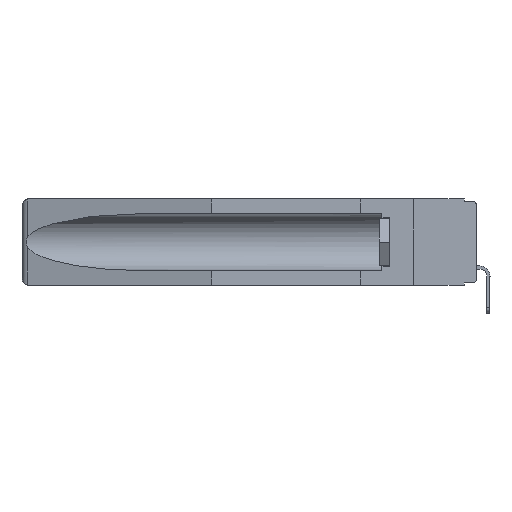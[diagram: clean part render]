
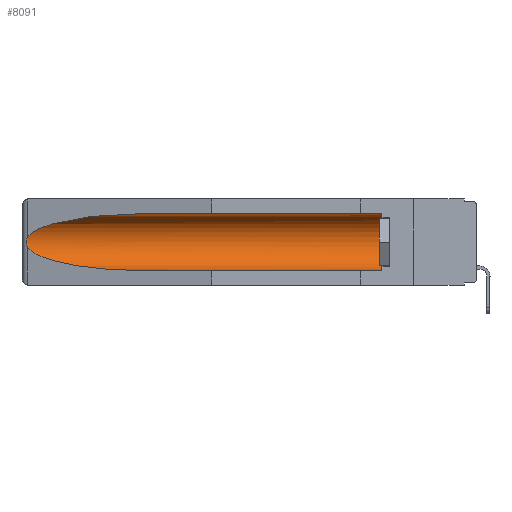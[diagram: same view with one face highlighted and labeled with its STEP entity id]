
A CAD part, left-side view. The second image highlights one B-rep face of the part: STEP entity #8091.
In plain terms, the highlighted cylindrical face has radius 2.857 mm (diameter 5.715 mm), a partial arc.
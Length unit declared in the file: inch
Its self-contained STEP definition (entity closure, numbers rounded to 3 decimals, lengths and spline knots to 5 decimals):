
#86 = CARTESIAN_POINT ( 'NONE',  ( 0.26537, 1.52718, -0.14972 ) ) ;
#136 = CARTESIAN_POINT ( 'NONE',  ( 0.2673, 1.5327, -0.16383 ) ) ;
#172 = EDGE_CURVE ( 'NONE', #9058, #12660, #3271, .T. ) ;
#1187 = DIRECTION ( 'NONE',  ( 0., 1., 0. ) ) ;
#1372 = DIRECTION ( 'NONE',  ( 0., 1., 0. ) ) ;
#1738 = CARTESIAN_POINT ( 'NONE',  ( 0.2673, 1.53269, -0.17917 ) ) ;
#1759 = ORIENTED_EDGE ( 'NONE', *, *, #14701, .T. ) ;
#1830 = CARTESIAN_POINT ( 'NONE',  ( 0.26654, 1.53092, -0.15636 ) ) ;
#1890 = CARTESIAN_POINT ( 'NONE',  ( 0.21114, 1.30732, -0.284 ) ) ;
#2155 = LINE ( 'NONE', #8612, #16605 ) ;
#2253 = EDGE_LOOP ( 'NONE', ( #1759, #11903, #10346, #12034, #5680, #13302 ) ) ;
#2475 = CARTESIAN_POINT ( 'NONE',  ( 0.155, -0.30754, -0.1715 ) ) ;
#3074 = EDGE_CURVE ( 'NONE', #16322, #10199, #15776, .T. ) ;
#3271 = LINE ( 'NONE', #19186, #10555 ) ;
#4268 = CARTESIAN_POINT ( 'NONE',  ( 0.155, 0.126, -0.1715 ) ) ;
#4823 = CARTESIAN_POINT ( 'NONE',  ( 0.26537, 1.52718, -0.19328 ) ) ;
#5309 = CARTESIAN_POINT ( 'NONE',  ( 0.155, 1.07973, -0.059 ) ) ;
#5680 = ORIENTED_EDGE ( 'NONE', *, *, #5923, .T. ) ;
#5923 = EDGE_CURVE ( 'NONE', #13357, #9058, #12169, .T. ) ;
#6426 = CARTESIAN_POINT ( 'NONE',  ( 0.155, 1.07973, -0.284 ) ) ;
#6949 = CARTESIAN_POINT ( 'NONE',  ( 0.155, 0.126, -0.059 ) ) ;
#8091 = ADVANCED_FACE ( 'NONE', ( #18598 ), #10551, .F. ) ;
#8191 = CARTESIAN_POINT ( 'NONE',  ( 0.26655, 1.53094, -0.18657 ) ) ;
#8358 = CARTESIAN_POINT ( 'NONE',  ( 0.155, 1.07973, -0.284 ) ) ;
#8612 = CARTESIAN_POINT ( 'NONE',  ( 0.155, -0.30754, -0.284 ) ) ;
#9058 = VERTEX_POINT ( 'NONE', #6949 ) ;
#9150 = DIRECTION ( 'NONE',  ( 0., 0., 1. ) ) ;
#9908 = CARTESIAN_POINT ( 'NONE',  ( 0.2675, 1.53308, -0.16763 ) ) ;
#10199 = VERTEX_POINT ( 'NONE', #6426 ) ;
#10346 = ORIENTED_EDGE ( 'NONE', *, *, #3074, .T. ) ;
#10551 = CYLINDRICAL_SURFACE ( 'NONE', #20017, 0.1125 ) ;
#10555 = VECTOR ( 'NONE', #1372, 39.37008 ) ;
#11758 = CARTESIAN_POINT ( 'NONE',  ( 0.155, 1.07973, -0.059 ) ) ;
#11903 = ORIENTED_EDGE ( 'NONE', *, *, #19838, .T. ) ;
#12034 = ORIENTED_EDGE ( 'NONE', *, *, #20011, .F. ) ;
#12169 = CIRCLE ( 'NONE', #16913, 0.1125 ) ;
#12452 = DIRECTION ( 'NONE',  ( 0., -1., 0. ) ) ;
#12660 = VERTEX_POINT ( 'NONE', #5309 ) ;
#12694 =( BOUNDED_CURVE ( )  B_SPLINE_CURVE ( 3, ( #11758, #18221, #14652, #86 ),
 .UNSPECIFIED., .F., .F. ) 
 B_SPLINE_CURVE_WITH_KNOTS ( ( 4, 4 ),
 ( 4.71239, 6.08839 ),
 .UNSPECIFIED. ) 
 CURVE ( )  GEOMETRIC_REPRESENTATION_ITEM ( )  RATIONAL_B_SPLINE_CURVE ( ( 1., 0.848, 0.848, 1. ) ) 
 REPRESENTATION_ITEM ( '' )  );
#13019 = CARTESIAN_POINT ( 'NONE',  ( 0.26537, 1.52718, -0.14972 ) ) ;
#13081 = CARTESIAN_POINT ( 'NONE',  ( 0.26537, 1.52718, -0.19328 ) ) ;
#13302 = ORIENTED_EDGE ( 'NONE', *, *, #172, .T. ) ;
#13357 = VERTEX_POINT ( 'NONE', #20550 ) ;
#14055 = DIRECTION ( 'NONE',  ( 0., 0., 1. ) ) ;
#14652 = CARTESIAN_POINT ( 'NONE',  ( 0.25451, 1.48313, -0.09465 ) ) ;
#14701 = EDGE_CURVE ( 'NONE', #12660, #19686, #12694, .T. ) ;
#14705 = CARTESIAN_POINT ( 'NONE',  ( 0.26597, 1.5296, -0.19026 ) ) ;
#14715 = B_SPLINE_CURVE_WITH_KNOTS ( 'NONE', 3,
 ( #13019, #16302, #1830, #136, #9908, #19350, #1738, #8191, #14705, #4823 ),
 .UNSPECIFIED., .F., .F.,
 ( 4, 2, 2, 2, 4 ),
 ( 0., 0.00029, 0.00058, 0.00087, 0.00117 ),
 .UNSPECIFIED. ) ;
#15776 =( BOUNDED_CURVE ( )  B_SPLINE_CURVE ( 3, ( #17558, #16469, #1890, #8358 ),
 .UNSPECIFIED., .F., .F. ) 
 B_SPLINE_CURVE_WITH_KNOTS ( ( 4, 4 ),
 ( 0.1948, 1.5708 ),
 .UNSPECIFIED. ) 
 CURVE ( )  GEOMETRIC_REPRESENTATION_ITEM ( )  RATIONAL_B_SPLINE_CURVE ( ( 1., 0.848, 0.848, 1. ) ) 
 REPRESENTATION_ITEM ( '' )  );
#16302 = CARTESIAN_POINT ( 'NONE',  ( 0.26597, 1.52961, -0.15275 ) ) ;
#16322 = VERTEX_POINT ( 'NONE', #13081 ) ;
#16469 = CARTESIAN_POINT ( 'NONE',  ( 0.25451, 1.48313, -0.24835 ) ) ;
#16605 = VECTOR ( 'NONE', #17127, 39.37008 ) ;
#16913 = AXIS2_PLACEMENT_3D ( 'NONE', #4268, #12452, #14055 ) ;
#17127 = DIRECTION ( 'NONE',  ( 0., 1., 0. ) ) ;
#17464 = CARTESIAN_POINT ( 'NONE',  ( 0.26537, 1.52718, -0.14972 ) ) ;
#17558 = CARTESIAN_POINT ( 'NONE',  ( 0.26537, 1.52718, -0.19328 ) ) ;
#18221 = CARTESIAN_POINT ( 'NONE',  ( 0.21114, 1.30732, -0.059 ) ) ;
#18598 = FACE_OUTER_BOUND ( 'NONE', #2253, .T. ) ;
#19186 = CARTESIAN_POINT ( 'NONE',  ( 0.155, -0.30754, -0.059 ) ) ;
#19350 = CARTESIAN_POINT ( 'NONE',  ( 0.2675, 1.53308, -0.17534 ) ) ;
#19686 = VERTEX_POINT ( 'NONE', #17464 ) ;
#19838 = EDGE_CURVE ( 'NONE', #19686, #16322, #14715, .T. ) ;
#20011 = EDGE_CURVE ( 'NONE', #13357, #10199, #2155, .T. ) ;
#20017 = AXIS2_PLACEMENT_3D ( 'NONE', #2475, #1187, #9150 ) ;
#20550 = CARTESIAN_POINT ( 'NONE',  ( 0.155, 0.126, -0.284 ) ) ;
